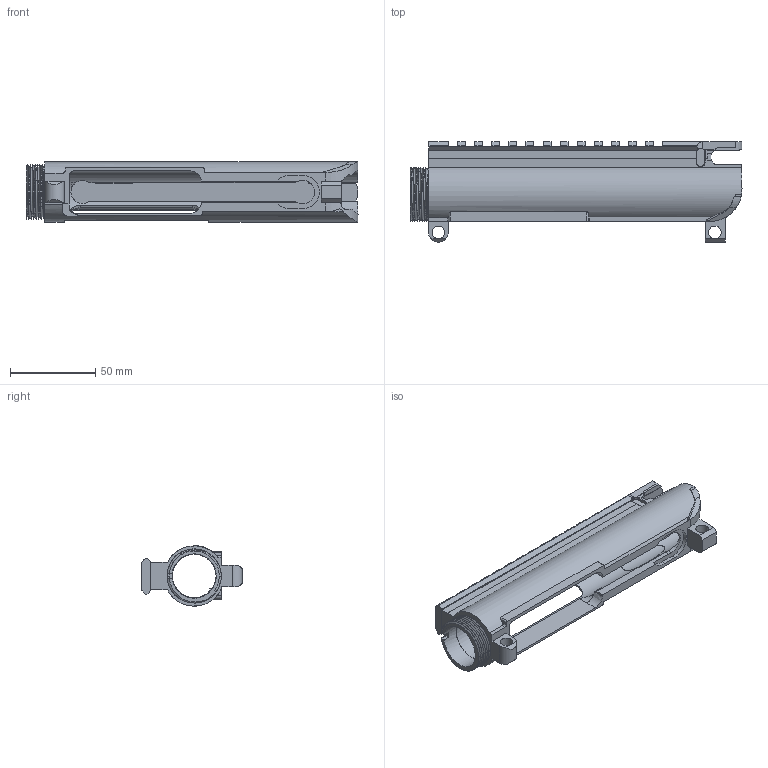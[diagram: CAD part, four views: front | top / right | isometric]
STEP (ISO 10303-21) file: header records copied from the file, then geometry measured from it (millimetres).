
FILE_DESCRIPTION(/* description */ (''),/* implementation_level */ '2;1');
FILE_NAME(/* name */ 'Upper Reciever - Daichi.step',/* time_stamp */ '2020-12-11T01:51:29-05:00',/* author */ (''),/* organization */ (''),/* preprocessor_version */ 'ST-DEVELOPER v18.1',/* originating_system */ 'Autodesk Translation Framework v9.7.1.1290',/* authorisation */ '');
FILE_SCHEMA (('AUTOMOTIVE_DESIGN { 1 0 10303 214 3 1 1 }'));
Length unit declared in the file: millimetre
Products named in the file (1): Upper Reciever - Daichi
Bounding box: 194.4 x 59 x 35.23 mm (x, y, z)
Volume: 78496 mm3; surface area: 49020.7 mm2
Topology: 1 solids, 2 shells, 398 faces, 1149 edges, 753 vertices
Faces by surface type: plane 239, cylinder 89, cone 52, bspline 15, torus 3
Full cylindrical faces by diameter (mm): 7.35 x1, 7.358 x1, 25.546 x1, 25.927 x1, 29.782 x1, 31.7 x4
Entity records: 15678 total; most frequent: CARTESIAN_POINT 5458, ORIENTED_EDGE 2296, DIRECTION 1912, EDGE_CURVE 1148, VERTEX_POINT 753, LINE 744, VECTOR 744, AXIS2_PLACEMENT_3D 584
